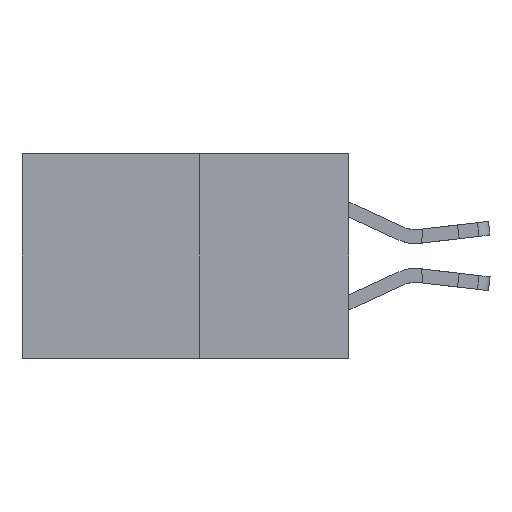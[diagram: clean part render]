
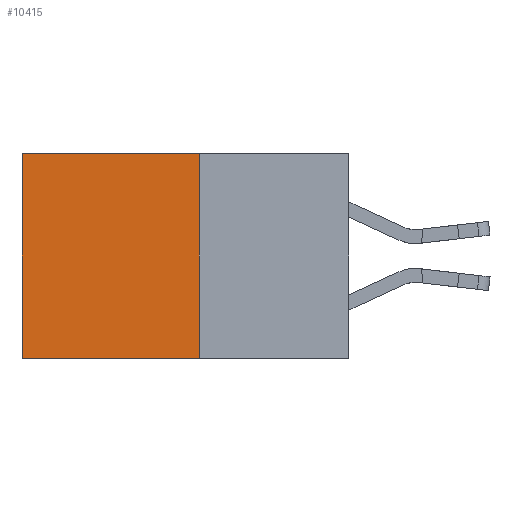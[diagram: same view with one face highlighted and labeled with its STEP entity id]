
A CAD part, left-side view. The second image highlights one B-rep face of the part: STEP entity #10415.
In plain terms, the highlighted planar face has unit normal (-1, 0, 0).
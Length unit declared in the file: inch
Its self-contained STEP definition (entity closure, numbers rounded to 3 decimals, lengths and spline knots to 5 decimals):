
#301 = EDGE_LOOP ( 'NONE', ( #13828, #13677, #13419, #12848 ) ) ;
#317 = LINE ( 'NONE', #418, #5955 ) ;
#418 = CARTESIAN_POINT ( 'NONE',  ( 0.277, 0.27, -0.37 ) ) ;
#429 = DIRECTION ( 'NONE',  ( 0., 1., 0. ) ) ;
#458 = CARTESIAN_POINT ( 'NONE',  ( 0.277, 0.27, -0.37 ) ) ;
#1119 = DIRECTION ( 'NONE',  ( 0., 1., 0. ) ) ;
#1222 = VERTEX_POINT ( 'NONE', #1227 ) ;
#1227 = CARTESIAN_POINT ( 'NONE',  ( 0.277, 0.27, 0. ) ) ;
#1590 = DIRECTION ( 'NONE',  ( 1., 0., 0. ) ) ;
#1700 = VECTOR ( 'NONE', #1119, 39.37008 ) ;
#1822 = VECTOR ( 'NONE', #5949, 39.37008 ) ;
#2328 = VERTEX_POINT ( 'NONE', #6268 ) ;
#2497 = LINE ( 'NONE', #5118, #14019 ) ;
#2753 = EDGE_CURVE ( 'NONE', #1222, #13167, #2497, .T. ) ;
#4674 = LINE ( 'NONE', #9171, #1700 ) ;
#5118 = CARTESIAN_POINT ( 'NONE',  ( 0.277, 0.27, -0.37 ) ) ;
#5207 = CARTESIAN_POINT ( 'NONE',  ( 0.277, 0.59, 0. ) ) ;
#5868 = CARTESIAN_POINT ( 'NONE',  ( 0.277, 0.59, -0.37 ) ) ;
#5949 = DIRECTION ( 'NONE',  ( 0., 0., -1. ) ) ;
#5955 = VECTOR ( 'NONE', #429, 39.37008 ) ;
#6268 = CARTESIAN_POINT ( 'NONE',  ( 0.277, 0.59, -0.37 ) ) ;
#6578 = EDGE_CURVE ( 'NONE', #11209, #2328, #13393, .T. ) ;
#7170 = PLANE ( 'NONE',  #13074 ) ;
#8151 = EDGE_CURVE ( 'NONE', #13167, #2328, #317, .T. ) ;
#9171 = CARTESIAN_POINT ( 'NONE',  ( 0.277, 0.27, 0. ) ) ;
#9385 = DIRECTION ( 'NONE',  ( 0., 0., -1. ) ) ;
#9393 = EDGE_CURVE ( 'NONE', #1222, #11209, #4674, .T. ) ;
#10046 = FACE_OUTER_BOUND ( 'NONE', #301, .T. ) ;
#10415 = ADVANCED_FACE ( 'NONE', ( #10046 ), #7170, .F. ) ;
#11209 = VERTEX_POINT ( 'NONE', #5207 ) ;
#12848 = ORIENTED_EDGE ( 'NONE', *, *, #9393, .T. ) ;
#13074 = AXIS2_PLACEMENT_3D ( 'NONE', #458, #1590, #9385 ) ;
#13089 = DIRECTION ( 'NONE',  ( 0., 0., -1. ) ) ;
#13167 = VERTEX_POINT ( 'NONE', #13573 ) ;
#13393 = LINE ( 'NONE', #5868, #1822 ) ;
#13419 = ORIENTED_EDGE ( 'NONE', *, *, #2753, .F. ) ;
#13573 = CARTESIAN_POINT ( 'NONE',  ( 0.277, 0.27, -0.37 ) ) ;
#13677 = ORIENTED_EDGE ( 'NONE', *, *, #8151, .F. ) ;
#13828 = ORIENTED_EDGE ( 'NONE', *, *, #6578, .T. ) ;
#14019 = VECTOR ( 'NONE', #13089, 39.37008 ) ;
